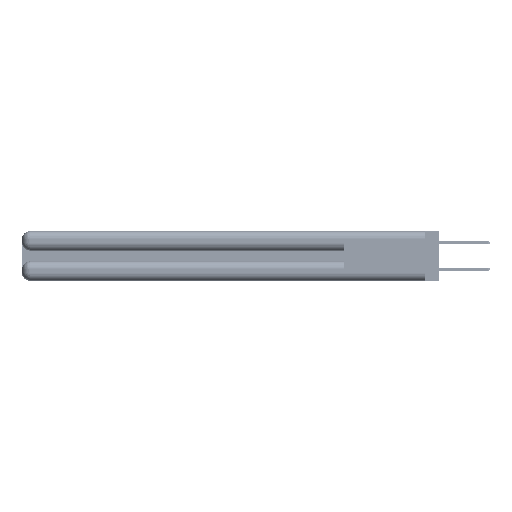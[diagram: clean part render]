
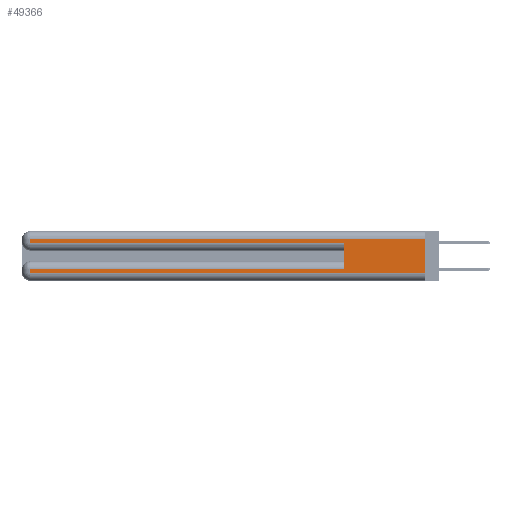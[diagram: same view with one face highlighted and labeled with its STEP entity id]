
A CAD part, left-side view. The second image highlights one B-rep face of the part: STEP entity #49366.
In plain terms, the highlighted planar face has unit normal (-1, 0, 0).
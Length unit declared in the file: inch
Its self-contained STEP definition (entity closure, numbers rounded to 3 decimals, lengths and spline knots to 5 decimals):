
#1249 = ORIENTED_EDGE ( 'NONE', *, *, #38741, .F. ) ;
#2069 = VECTOR ( 'NONE', #37830, 39.37008 ) ;
#3706 = VECTOR ( 'NONE', #25558, 39.37008 ) ;
#4073 = CARTESIAN_POINT ( 'NONE',  ( 0., 2.94, 0.085 ) ) ;
#4456 = LINE ( 'NONE', #45105, #5743 ) ;
#5151 = VERTEX_POINT ( 'NONE', #30009 ) ;
#5164 = EDGE_LOOP ( 'NONE', ( #1249, #41962, #35865, #25871, #45262, #36160, #48738, #25314 ) ) ;
#5743 = VECTOR ( 'NONE', #45795, 39.37008 ) ;
#5934 = EDGE_CURVE ( 'NONE', #11992, #15969, #45124, .T. ) ;
#6480 = CARTESIAN_POINT ( 'NONE',  ( 0., 0., 0.06 ) ) ;
#6872 = VERTEX_POINT ( 'NONE', #4073 ) ;
#8556 = CARTESIAN_POINT ( 'NONE',  ( 0., 0.6, 0.085 ) ) ;
#8755 = CARTESIAN_POINT ( 'NONE',  ( 0., 2.94, 0.285 ) ) ;
#8818 = CARTESIAN_POINT ( 'NONE',  ( 0., 0., 0.06 ) ) ;
#9352 = VECTOR ( 'NONE', #15077, 39.37008 ) ;
#10375 = PLANE ( 'NONE',  #22095 ) ;
#10750 = CARTESIAN_POINT ( 'NONE',  ( 0., 0.6, 0.145 ) ) ;
#10967 = CARTESIAN_POINT ( 'NONE',  ( 0., 0., 0.31 ) ) ;
#11215 = LINE ( 'NONE', #10967, #9352 ) ;
#11992 = VERTEX_POINT ( 'NONE', #8556 ) ;
#15077 = DIRECTION ( 'NONE',  ( 0., 1., 0. ) ) ;
#15450 = CARTESIAN_POINT ( 'NONE',  ( 0., 0., 0.37 ) ) ;
#15969 = VERTEX_POINT ( 'NONE', #32173 ) ;
#17883 = DIRECTION ( 'NONE',  ( 0., -1., 0. ) ) ;
#18939 = DIRECTION ( 'NONE',  ( 0., 0., 1. ) ) ;
#19240 = EDGE_CURVE ( 'NONE', #40598, #15969, #40574, .T. ) ;
#22095 = AXIS2_PLACEMENT_3D ( 'NONE', #46801, #26775, #22484 ) ;
#22484 = DIRECTION ( 'NONE',  ( 0., 0., -1. ) ) ;
#22821 = LINE ( 'NONE', #8818, #3706 ) ;
#25314 = ORIENTED_EDGE ( 'NONE', *, *, #40042, .T. ) ;
#25558 = DIRECTION ( 'NONE',  ( 0., -1., 0. ) ) ;
#25596 = EDGE_CURVE ( 'NONE', #11992, #6872, #50395, .T. ) ;
#25871 = ORIENTED_EDGE ( 'NONE', *, *, #19240, .T. ) ;
#26516 = CARTESIAN_POINT ( 'NONE',  ( 0., 2.94, 0.31 ) ) ;
#26775 = DIRECTION ( 'NONE',  ( 1., 0., 0. ) ) ;
#29255 = VECTOR ( 'NONE', #18939, 39.37008 ) ;
#29373 = DIRECTION ( 'NONE',  ( 0., 0., -1. ) ) ;
#30009 = CARTESIAN_POINT ( 'NONE',  ( 0., 2.94, 0.06 ) ) ;
#32173 = CARTESIAN_POINT ( 'NONE',  ( 0., 0.6, 0.285 ) ) ;
#32210 = LINE ( 'NONE', #49748, #45551 ) ;
#32531 = EDGE_CURVE ( 'NONE', #33986, #40598, #32210, .T. ) ;
#33986 = VERTEX_POINT ( 'NONE', #26516 ) ;
#35865 = ORIENTED_EDGE ( 'NONE', *, *, #32531, .T. ) ;
#36019 = FACE_OUTER_BOUND ( 'NONE', #5164, .T. ) ;
#36160 = ORIENTED_EDGE ( 'NONE', *, *, #25596, .T. ) ;
#36763 = CARTESIAN_POINT ( 'NONE',  ( 0., 0., 0.285 ) ) ;
#37215 = CARTESIAN_POINT ( 'NONE',  ( 0., 0., 0.31 ) ) ;
#37830 = DIRECTION ( 'NONE',  ( 0., 1., 0. ) ) ;
#38741 = EDGE_CURVE ( 'NONE', #47168, #39201, #43459, .T. ) ;
#39201 = VERTEX_POINT ( 'NONE', #6480 ) ;
#40042 = EDGE_CURVE ( 'NONE', #5151, #39201, #22821, .T. ) ;
#40574 = LINE ( 'NONE', #36763, #44362 ) ;
#40598 = VERTEX_POINT ( 'NONE', #8755 ) ;
#41024 = CARTESIAN_POINT ( 'NONE',  ( 0., 0., 0.085 ) ) ;
#41962 = ORIENTED_EDGE ( 'NONE', *, *, #48395, .T. ) ;
#43459 = LINE ( 'NONE', #15450, #49819 ) ;
#44362 = VECTOR ( 'NONE', #17883, 39.37008 ) ;
#44532 = EDGE_CURVE ( 'NONE', #6872, #5151, #4456, .T. ) ;
#45105 = CARTESIAN_POINT ( 'NONE',  ( 0., 2.94, 0.37 ) ) ;
#45124 = LINE ( 'NONE', #10750, #29255 ) ;
#45262 = ORIENTED_EDGE ( 'NONE', *, *, #5934, .F. ) ;
#45551 = VECTOR ( 'NONE', #29373, 39.37008 ) ;
#45795 = DIRECTION ( 'NONE',  ( 0., 0., -1. ) ) ;
#46801 = CARTESIAN_POINT ( 'NONE',  ( 0., 0., 0.37 ) ) ;
#47168 = VERTEX_POINT ( 'NONE', #37215 ) ;
#48395 = EDGE_CURVE ( 'NONE', #47168, #33986, #11215, .T. ) ;
#48738 = ORIENTED_EDGE ( 'NONE', *, *, #44532, .T. ) ;
#49366 = ADVANCED_FACE ( 'NONE', ( #36019 ), #10375, .F. ) ;
#49748 = CARTESIAN_POINT ( 'NONE',  ( 0., 2.94, 0.37 ) ) ;
#49819 = VECTOR ( 'NONE', #52001, 39.37008 ) ;
#50395 = LINE ( 'NONE', #41024, #2069 ) ;
#52001 = DIRECTION ( 'NONE',  ( 0., 0., -1. ) ) ;
